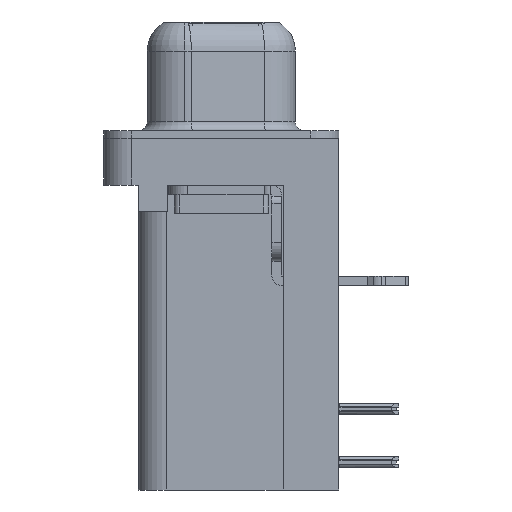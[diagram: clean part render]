
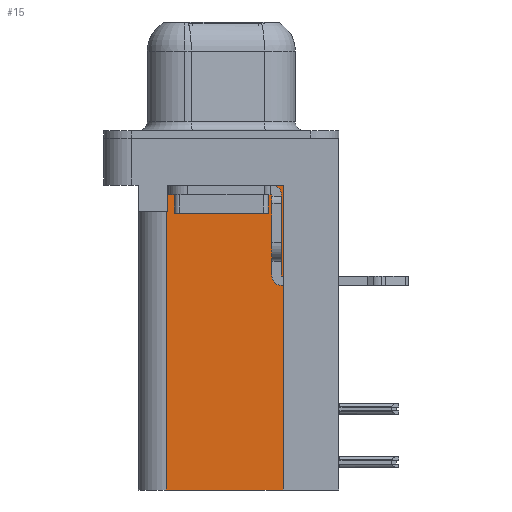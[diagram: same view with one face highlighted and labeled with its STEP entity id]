
A CAD part, left-side view. The second image highlights one B-rep face of the part: STEP entity #15.
In plain terms, the highlighted planar face has unit normal (-1, 0, 0).
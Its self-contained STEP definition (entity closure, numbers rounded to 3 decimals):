
#15 = ADVANCED_FACE ( 'NONE', ( #22599 ), #30213, .F. ) ;
#1006 = EDGE_CURVE ( 'NONE', #14347, #7707, #16630, .T. ) ;
#1632 = CARTESIAN_POINT ( 'NONE',  ( 3.7, -3.295, -2.5 ) ) ;
#2958 = DIRECTION ( 'NONE',  ( 0., 1., 0. ) ) ;
#3215 = DIRECTION ( 'NONE',  ( 0., 1., 0. ) ) ;
#4124 = DIRECTION ( 'NONE',  ( 0., 0., 1. ) ) ;
#4503 = ORIENTED_EDGE ( 'NONE', *, *, #31129, .T. ) ;
#7016 = CARTESIAN_POINT ( 'NONE',  ( 3.7, 2.895, -3.9 ) ) ;
#7225 = CARTESIAN_POINT ( 'NONE',  ( 3.7, 2.925, -18.76 ) ) ;
#7231 = VERTEX_POINT ( 'NONE', #7554 ) ;
#7554 = CARTESIAN_POINT ( 'NONE',  ( 3.7, 2.895, -3.9 ) ) ;
#7707 = VERTEX_POINT ( 'NONE', #7225 ) ;
#8628 = CARTESIAN_POINT ( 'NONE',  ( 3.7, 2.925, -18.76 ) ) ;
#8760 = VERTEX_POINT ( 'NONE', #30834 ) ;
#8850 = ORIENTED_EDGE ( 'NONE', *, *, #28036, .T. ) ;
#9429 = VERTEX_POINT ( 'NONE', #29171 ) ;
#10555 = CARTESIAN_POINT ( 'NONE',  ( 3.7, -3.295, -18.76 ) ) ;
#11688 = DIRECTION ( 'NONE',  ( 0., 1., 0. ) ) ;
#12044 = VECTOR ( 'NONE', #19398, 1000. ) ;
#13731 = ORIENTED_EDGE ( 'NONE', *, *, #18964, .T. ) ;
#14347 = VERTEX_POINT ( 'NONE', #26500 ) ;
#14935 = EDGE_LOOP ( 'NONE', ( #23393, #13731, #8850, #25491, #19440, #4503 ) ) ;
#16630 = LINE ( 'NONE', #10555, #16965 ) ;
#16965 = VECTOR ( 'NONE', #11688, 1000. ) ;
#17685 = EDGE_CURVE ( 'NONE', #23535, #8760, #26404, .T. ) ;
#18964 = EDGE_CURVE ( 'NONE', #8760, #7231, #30815, .T. ) ;
#19398 = DIRECTION ( 'NONE',  ( 0., 0., -1. ) ) ;
#19440 = ORIENTED_EDGE ( 'NONE', *, *, #1006, .F. ) ;
#19853 = CARTESIAN_POINT ( 'NONE',  ( 3.7, 0., -3.9 ) ) ;
#20202 = LINE ( 'NONE', #30931, #20391 ) ;
#20391 = VECTOR ( 'NONE', #4124, 1000. ) ;
#20496 = EDGE_CURVE ( 'NONE', #7707, #9429, #26628, .T. ) ;
#20762 = DIRECTION ( 'NONE',  ( 0., 1., 0. ) ) ;
#22599 = FACE_OUTER_BOUND ( 'NONE', #14935, .T. ) ;
#22645 = AXIS2_PLACEMENT_3D ( 'NONE', #30998, #30937, #3215 ) ;
#23393 = ORIENTED_EDGE ( 'NONE', *, *, #17685, .T. ) ;
#23535 = VERTEX_POINT ( 'NONE', #1632 ) ;
#25491 = ORIENTED_EDGE ( 'NONE', *, *, #20496, .F. ) ;
#26311 = VECTOR ( 'NONE', #20762, 1000. ) ;
#26404 = LINE ( 'NONE', #28141, #26311 ) ;
#26500 = CARTESIAN_POINT ( 'NONE',  ( 3.7, -3.295, -18.76 ) ) ;
#26628 = LINE ( 'NONE', #8628, #26692 ) ;
#26692 = VECTOR ( 'NONE', #28109, 1000. ) ;
#28036 = EDGE_CURVE ( 'NONE', #7231, #9429, #31021, .T. ) ;
#28109 = DIRECTION ( 'NONE',  ( 0., 0., 1. ) ) ;
#28141 = CARTESIAN_POINT ( 'NONE',  ( 3.7, -3.295, -2.5 ) ) ;
#29171 = CARTESIAN_POINT ( 'NONE',  ( 3.7, 2.925, -3.9 ) ) ;
#30213 = PLANE ( 'NONE',  #22645 ) ;
#30732 = VECTOR ( 'NONE', #2958, 1000. ) ;
#30815 = LINE ( 'NONE', #7016, #12044 ) ;
#30834 = CARTESIAN_POINT ( 'NONE',  ( 3.7, 2.895, -2.5 ) ) ;
#30931 = CARTESIAN_POINT ( 'NONE',  ( 3.7, -3.295, -18.76 ) ) ;
#30937 = DIRECTION ( 'NONE',  ( 1., 0., 0. ) ) ;
#30998 = CARTESIAN_POINT ( 'NONE',  ( 3.7, -3.295, -18.76 ) ) ;
#31021 = LINE ( 'NONE', #19853, #30732 ) ;
#31129 = EDGE_CURVE ( 'NONE', #14347, #23535, #20202, .T. ) ;
